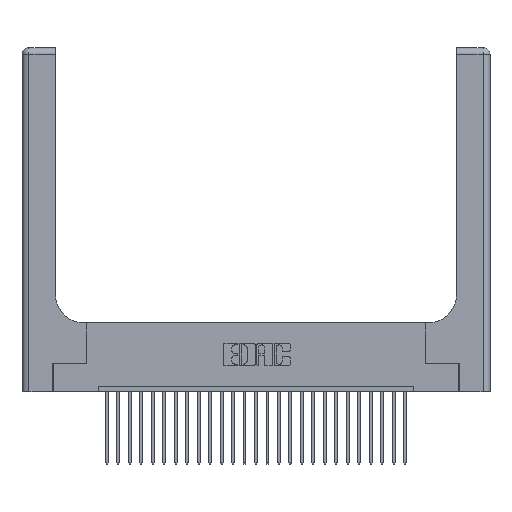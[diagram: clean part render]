
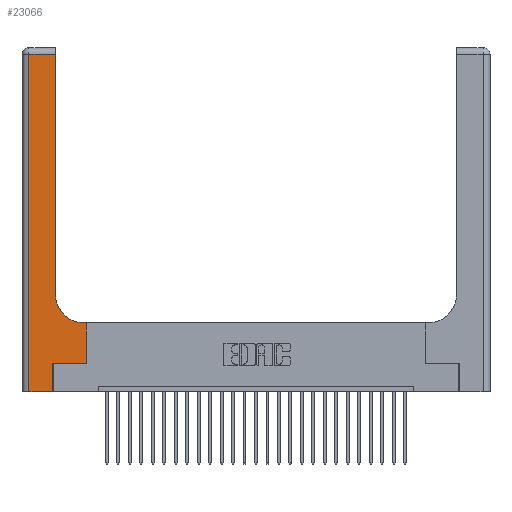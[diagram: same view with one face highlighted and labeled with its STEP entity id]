
A CAD part, top view. The second image highlights one B-rep face of the part: STEP entity #23066.
In plain terms, the highlighted planar face has unit normal (0, 0, 1).
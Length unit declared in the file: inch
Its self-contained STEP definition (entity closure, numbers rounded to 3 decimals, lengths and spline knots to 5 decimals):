
#388 = DIRECTION ( 'NONE',  ( 0., 1., 0. ) ) ;
#988 = CARTESIAN_POINT ( 'NONE',  ( 0.2915, 2.94, 0.37 ) ) ;
#1921 = CARTESIAN_POINT ( 'NONE',  ( 0.269, 0.25, 0.37 ) ) ;
#2413 = VERTEX_POINT ( 'NONE', #3526 ) ;
#2507 = ORIENTED_EDGE ( 'NONE', *, *, #3824, .T. ) ;
#2735 = DIRECTION ( 'NONE',  ( -1., 0., 0. ) ) ;
#3507 = EDGE_CURVE ( 'NONE', #16177, #5400, #4138, .T. ) ;
#3526 = CARTESIAN_POINT ( 'NONE',  ( 0.269, 0.25, 0.37 ) ) ;
#3824 = EDGE_CURVE ( 'NONE', #25475, #2413, #17702, .T. ) ;
#3859 = EDGE_CURVE ( 'NONE', #16760, #19523, #10422, .T. ) ;
#3861 = LINE ( 'NONE', #16075, #17439 ) ;
#4138 = LINE ( 'NONE', #23597, #13403 ) ;
#4160 = CARTESIAN_POINT ( 'NONE',  ( 0.5585, 0.6, 0.37 ) ) ;
#4324 = EDGE_CURVE ( 'NONE', #5400, #20560, #16353, .T. ) ;
#4548 = ORIENTED_EDGE ( 'NONE', *, *, #4324, .T. ) ;
#4754 = VECTOR ( 'NONE', #15883, 39.37008 ) ;
#5245 = CIRCLE ( 'NONE', #20618, 0.25 ) ;
#5400 = VERTEX_POINT ( 'NONE', #4160 ) ;
#5807 = DIRECTION ( 'NONE',  ( 0., 0., -1. ) ) ;
#5902 = DIRECTION ( 'NONE',  ( 0., -1., 0. ) ) ;
#6229 = DIRECTION ( 'NONE',  ( 1., 0., 0. ) ) ;
#7435 = DIRECTION ( 'NONE',  ( 0., 1., 0. ) ) ;
#8431 = EDGE_CURVE ( 'NONE', #16354, #16760, #3861, .T. ) ;
#8682 = ORIENTED_EDGE ( 'NONE', *, *, #8431, .T. ) ;
#9100 = LINE ( 'NONE', #27157, #24054 ) ;
#10422 = LINE ( 'NONE', #14241, #4754 ) ;
#10909 = PLANE ( 'NONE',  #26817 ) ;
#11005 = CARTESIAN_POINT ( 'NONE',  ( 0.5415, 0.6, 0.37 ) ) ;
#11083 = VECTOR ( 'NONE', #22683, 39.37008 ) ;
#11177 = EDGE_CURVE ( 'NONE', #2413, #16177, #22228, .T. ) ;
#11584 = EDGE_CURVE ( 'NONE', #20560, #16354, #5245, .T. ) ;
#12396 = CARTESIAN_POINT ( 'NONE',  ( 0.06, 0., 0.37 ) ) ;
#13216 = CARTESIAN_POINT ( 'NONE',  ( 0., 3., 0.37 ) ) ;
#13320 = VECTOR ( 'NONE', #6229, 39.37008 ) ;
#13403 = VECTOR ( 'NONE', #388, 39.37008 ) ;
#13659 = EDGE_CURVE ( 'NONE', #19523, #16944, #9100, .T. ) ;
#14208 = CARTESIAN_POINT ( 'NONE',  ( 0.2915, 0.85, 0.37 ) ) ;
#14241 = CARTESIAN_POINT ( 'NONE',  ( 0., 2.94, 0.37 ) ) ;
#14448 = DIRECTION ( 'NONE',  ( 1., 0., 0. ) ) ;
#15463 = DIRECTION ( 'NONE',  ( 0., 0., -1. ) ) ;
#15852 = ORIENTED_EDGE ( 'NONE', *, *, #17486, .T. ) ;
#15883 = DIRECTION ( 'NONE',  ( -1., 0., 0. ) ) ;
#16075 = CARTESIAN_POINT ( 'NONE',  ( 0.2915, 3., 0.37 ) ) ;
#16177 = VERTEX_POINT ( 'NONE', #20091 ) ;
#16353 = LINE ( 'NONE', #24466, #26978 ) ;
#16354 = VERTEX_POINT ( 'NONE', #14208 ) ;
#16662 = FACE_OUTER_BOUND ( 'NONE', #23680, .T. ) ;
#16729 = ORIENTED_EDGE ( 'NONE', *, *, #13659, .T. ) ;
#16760 = VERTEX_POINT ( 'NONE', #988 ) ;
#16944 = VERTEX_POINT ( 'NONE', #12396 ) ;
#17439 = VECTOR ( 'NONE', #7435, 39.37008 ) ;
#17486 = EDGE_CURVE ( 'NONE', #16944, #25475, #19959, .T. ) ;
#17702 = LINE ( 'NONE', #20726, #11083 ) ;
#17982 = ORIENTED_EDGE ( 'NONE', *, *, #11177, .T. ) ;
#18508 = DIRECTION ( 'NONE',  ( -1., 0., 0. ) ) ;
#18619 = ORIENTED_EDGE ( 'NONE', *, *, #11584, .T. ) ;
#18847 = CARTESIAN_POINT ( 'NONE',  ( 0., 0., 0.37 ) ) ;
#19523 = VERTEX_POINT ( 'NONE', #21625 ) ;
#19959 = LINE ( 'NONE', #18847, #13320 ) ;
#20091 = CARTESIAN_POINT ( 'NONE',  ( 0.5585, 0.25, 0.37 ) ) ;
#20560 = VERTEX_POINT ( 'NONE', #11005 ) ;
#20618 = AXIS2_PLACEMENT_3D ( 'NONE', #25006, #5807, #14448 ) ;
#20726 = CARTESIAN_POINT ( 'NONE',  ( 0.269, 0., 0.37 ) ) ;
#21625 = CARTESIAN_POINT ( 'NONE',  ( 0.06, 2.94, 0.37 ) ) ;
#22228 = LINE ( 'NONE', #1921, #23847 ) ;
#22683 = DIRECTION ( 'NONE',  ( 0., 1., 0. ) ) ;
#23066 = ADVANCED_FACE ( 'NONE', ( #16662 ), #10909, .F. ) ;
#23597 = CARTESIAN_POINT ( 'NONE',  ( 0.5585, 0.25, 0.37 ) ) ;
#23680 = EDGE_LOOP ( 'NONE', ( #8682, #24561, #16729, #15852, #2507, #17982, #24679, #4548, #18619 ) ) ;
#23808 = DIRECTION ( 'NONE',  ( 1., 0., 0. ) ) ;
#23847 = VECTOR ( 'NONE', #23808, 39.37008 ) ;
#23856 = CARTESIAN_POINT ( 'NONE',  ( 0.269, 0., 0.37 ) ) ;
#24054 = VECTOR ( 'NONE', #5902, 39.37008 ) ;
#24466 = CARTESIAN_POINT ( 'NONE',  ( 0.2915, 0.6, 0.37 ) ) ;
#24561 = ORIENTED_EDGE ( 'NONE', *, *, #3859, .T. ) ;
#24679 = ORIENTED_EDGE ( 'NONE', *, *, #3507, .T. ) ;
#25006 = CARTESIAN_POINT ( 'NONE',  ( 0.5415, 0.85, 0.37 ) ) ;
#25475 = VERTEX_POINT ( 'NONE', #23856 ) ;
#26817 = AXIS2_PLACEMENT_3D ( 'NONE', #13216, #15463, #2735 ) ;
#26978 = VECTOR ( 'NONE', #18508, 39.37008 ) ;
#27157 = CARTESIAN_POINT ( 'NONE',  ( 0.06, 3., 0.37 ) ) ;
